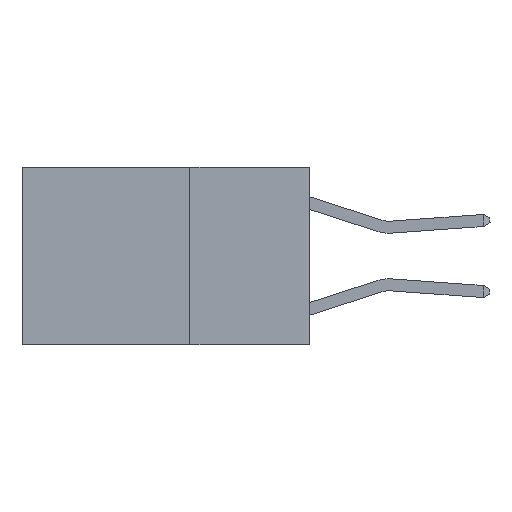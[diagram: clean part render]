
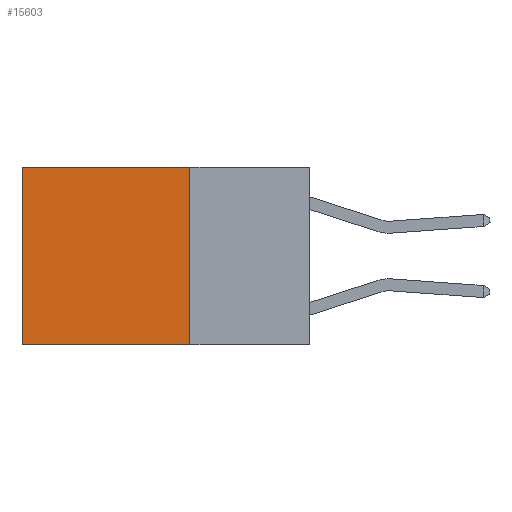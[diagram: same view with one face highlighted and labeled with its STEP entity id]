
A CAD part, left-side view. The second image highlights one B-rep face of the part: STEP entity #15603.
In plain terms, the highlighted planar face has unit normal (-1, 0, 0).
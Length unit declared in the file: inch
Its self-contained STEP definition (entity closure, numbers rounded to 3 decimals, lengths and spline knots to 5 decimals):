
#445 = EDGE_CURVE ( 'NONE', #5083, #15049, #15674, .T. ) ;
#1013 = ORIENTED_EDGE ( 'NONE', *, *, #15359, .F. ) ;
#1113 = LINE ( 'NONE', #8061, #13709 ) ;
#1355 = DIRECTION ( 'NONE',  ( 0., 0., -1. ) ) ;
#1823 = VECTOR ( 'NONE', #6050, 39.37008 ) ;
#2359 = ORIENTED_EDGE ( 'NONE', *, *, #445, .F. ) ;
#2448 = VERTEX_POINT ( 'NONE', #8059 ) ;
#2460 = CARTESIAN_POINT ( 'NONE',  ( 0.2625, 0.25, 0. ) ) ;
#2577 = LINE ( 'NONE', #15230, #8950 ) ;
#2645 = CARTESIAN_POINT ( 'NONE',  ( 0.2625, 0.25, 0. ) ) ;
#3973 = ORIENTED_EDGE ( 'NONE', *, *, #5121, .T. ) ;
#4499 = CARTESIAN_POINT ( 'NONE',  ( 0.2625, 0.6, 0. ) ) ;
#4848 = LINE ( 'NONE', #13481, #1823 ) ;
#5083 = VERTEX_POINT ( 'NONE', #2645 ) ;
#5121 = EDGE_CURVE ( 'NONE', #5083, #6695, #2577, .T. ) ;
#6050 = DIRECTION ( 'NONE',  ( 0., 1., 0. ) ) ;
#6695 = VERTEX_POINT ( 'NONE', #4499 ) ;
#8059 = CARTESIAN_POINT ( 'NONE',  ( 0.2625, 0.6, -0.37 ) ) ;
#8061 = CARTESIAN_POINT ( 'NONE',  ( 0.2625, 0.6, 0. ) ) ;
#8950 = VECTOR ( 'NONE', #12746, 39.37008 ) ;
#9010 = DIRECTION ( 'NONE',  ( 1., 0., 0. ) ) ;
#9452 = AXIS2_PLACEMENT_3D ( 'NONE', #11407, #9010, #1355 ) ;
#9511 = VECTOR ( 'NONE', #11272, 39.37008 ) ;
#10622 = ORIENTED_EDGE ( 'NONE', *, *, #10985, .T. ) ;
#10985 = EDGE_CURVE ( 'NONE', #6695, #2448, #1113, .T. ) ;
#11272 = DIRECTION ( 'NONE',  ( 0., 0., -1. ) ) ;
#11407 = CARTESIAN_POINT ( 'NONE',  ( 0.2625, 0.25, 0. ) ) ;
#12746 = DIRECTION ( 'NONE',  ( 0., 1., 0. ) ) ;
#12897 = CARTESIAN_POINT ( 'NONE',  ( 0.2625, 0.25, -0.37 ) ) ;
#13295 = DIRECTION ( 'NONE',  ( 0., 0., -1. ) ) ;
#13481 = CARTESIAN_POINT ( 'NONE',  ( 0.2625, 0.25, -0.37 ) ) ;
#13709 = VECTOR ( 'NONE', #13295, 39.37008 ) ;
#13863 = EDGE_LOOP ( 'NONE', ( #10622, #1013, #2359, #3973 ) ) ;
#13893 = PLANE ( 'NONE',  #9452 ) ;
#14556 = FACE_OUTER_BOUND ( 'NONE', #13863, .T. ) ;
#15049 = VERTEX_POINT ( 'NONE', #12897 ) ;
#15230 = CARTESIAN_POINT ( 'NONE',  ( 0.2625, 0.25, 0. ) ) ;
#15359 = EDGE_CURVE ( 'NONE', #15049, #2448, #4848, .T. ) ;
#15603 = ADVANCED_FACE ( 'NONE', ( #14556 ), #13893, .F. ) ;
#15674 = LINE ( 'NONE', #2460, #9511 ) ;
